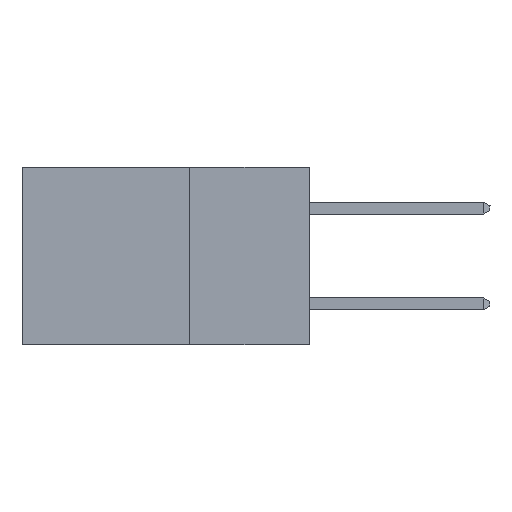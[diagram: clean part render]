
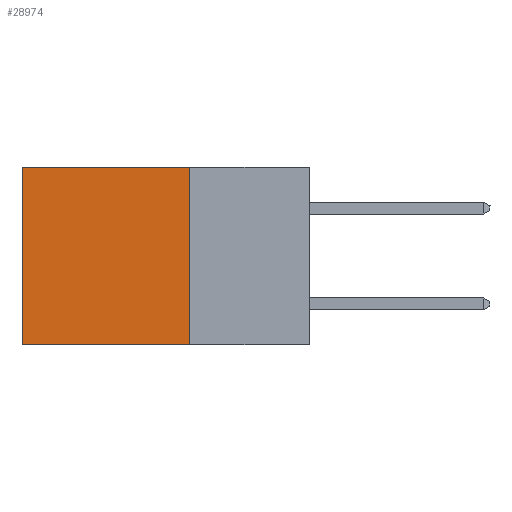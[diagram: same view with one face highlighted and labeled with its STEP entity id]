
A CAD part, left-side view. The second image highlights one B-rep face of the part: STEP entity #28974.
In plain terms, the highlighted planar face has unit normal (-1, 0, 0).
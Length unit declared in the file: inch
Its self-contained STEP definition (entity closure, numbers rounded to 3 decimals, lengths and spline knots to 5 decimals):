
#65 = EDGE_LOOP ( 'NONE', ( #25938, #14603, #9605, #1529 ) ) ;
#1529 = ORIENTED_EDGE ( 'NONE', *, *, #4899, .T. ) ;
#2806 = VECTOR ( 'NONE', #28013, 39.37008 ) ;
#4899 = EDGE_CURVE ( 'NONE', #32346, #25161, #29105, .T. ) ;
#5063 = CARTESIAN_POINT ( 'NONE',  ( 0.2875, 0.6, 0. ) ) ;
#8198 = VECTOR ( 'NONE', #17454, 39.37008 ) ;
#9590 = AXIS2_PLACEMENT_3D ( 'NONE', #32411, #12917, #15946 ) ;
#9605 = ORIENTED_EDGE ( 'NONE', *, *, #15007, .F. ) ;
#12917 = DIRECTION ( 'NONE',  ( 1., 0., 0. ) ) ;
#14603 = ORIENTED_EDGE ( 'NONE', *, *, #37575, .F. ) ;
#15002 = LINE ( 'NONE', #23692, #38729 ) ;
#15007 = EDGE_CURVE ( 'NONE', #32346, #17483, #32459, .T. ) ;
#15292 = LINE ( 'NONE', #15557, #31299 ) ;
#15557 = CARTESIAN_POINT ( 'NONE',  ( 0.2875, 0.25, -0.37 ) ) ;
#15946 = DIRECTION ( 'NONE',  ( 0., 0., -1. ) ) ;
#16094 = DIRECTION ( 'NONE',  ( 0., 1., 0. ) ) ;
#17454 = DIRECTION ( 'NONE',  ( 0., 0., -1. ) ) ;
#17483 = VERTEX_POINT ( 'NONE', #26057 ) ;
#20636 = FACE_OUTER_BOUND ( 'NONE', #65, .T. ) ;
#20824 = CARTESIAN_POINT ( 'NONE',  ( 0.2875, 0.25, 0. ) ) ;
#23332 = CARTESIAN_POINT ( 'NONE',  ( 0.2875, 0.25, 0. ) ) ;
#23692 = CARTESIAN_POINT ( 'NONE',  ( 0.2875, 0.6, 0. ) ) ;
#23753 = EDGE_CURVE ( 'NONE', #25161, #30195, #15002, .T. ) ;
#25161 = VERTEX_POINT ( 'NONE', #5063 ) ;
#25938 = ORIENTED_EDGE ( 'NONE', *, *, #23753, .T. ) ;
#26057 = CARTESIAN_POINT ( 'NONE',  ( 0.2875, 0.25, -0.37 ) ) ;
#28013 = DIRECTION ( 'NONE',  ( 0., 1., 0. ) ) ;
#28974 = ADVANCED_FACE ( 'NONE', ( #20636 ), #42462, .F. ) ;
#29105 = LINE ( 'NONE', #30478, #2806 ) ;
#30195 = VERTEX_POINT ( 'NONE', #32308 ) ;
#30435 = DIRECTION ( 'NONE',  ( 0., 0., -1. ) ) ;
#30478 = CARTESIAN_POINT ( 'NONE',  ( 0.2875, 0.25, 0. ) ) ;
#31299 = VECTOR ( 'NONE', #16094, 39.37008 ) ;
#32308 = CARTESIAN_POINT ( 'NONE',  ( 0.2875, 0.6, -0.37 ) ) ;
#32346 = VERTEX_POINT ( 'NONE', #23332 ) ;
#32411 = CARTESIAN_POINT ( 'NONE',  ( 0.2875, 0.25, 0. ) ) ;
#32459 = LINE ( 'NONE', #20824, #8198 ) ;
#37575 = EDGE_CURVE ( 'NONE', #17483, #30195, #15292, .T. ) ;
#38729 = VECTOR ( 'NONE', #30435, 39.37008 ) ;
#42462 = PLANE ( 'NONE',  #9590 ) ;
